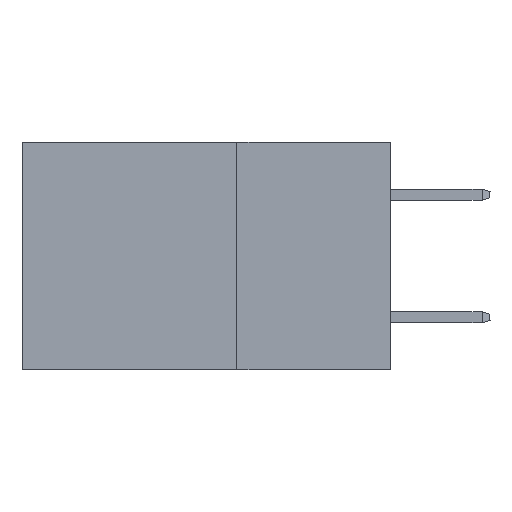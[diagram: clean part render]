
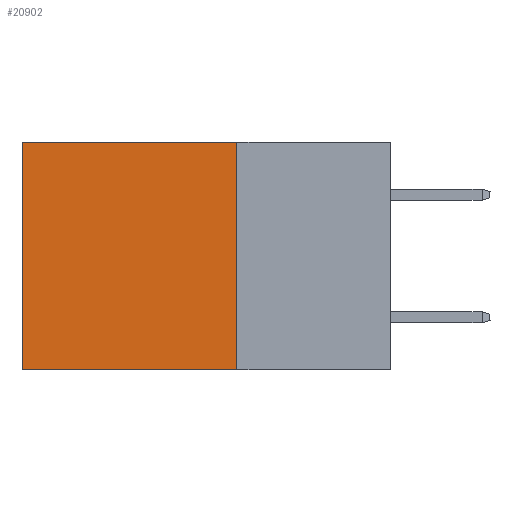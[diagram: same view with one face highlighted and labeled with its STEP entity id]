
A CAD part, left-side view. The second image highlights one B-rep face of the part: STEP entity #20902.
In plain terms, the highlighted planar face has unit normal (-1, 0, 0).
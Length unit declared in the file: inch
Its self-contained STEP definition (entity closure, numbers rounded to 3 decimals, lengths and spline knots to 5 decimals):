
#150 = CARTESIAN_POINT ( 'NONE',  ( 0.2875, 0.25, -0.37 ) ) ;
#2286 = DIRECTION ( 'NONE',  ( 0., 1., 0. ) ) ;
#2572 = DIRECTION ( 'NONE',  ( 0., 0., -1. ) ) ;
#2621 = ORIENTED_EDGE ( 'NONE', *, *, #12507, .T. ) ;
#3414 = VECTOR ( 'NONE', #31284, 39.37008 ) ;
#3448 = DIRECTION ( 'NONE',  ( 0., 0., -1. ) ) ;
#4628 = CARTESIAN_POINT ( 'NONE',  ( 0.2875, 0.6, -0.37 ) ) ;
#4707 = VECTOR ( 'NONE', #27309, 39.37008 ) ;
#4911 = VECTOR ( 'NONE', #2286, 39.37008 ) ;
#5128 = FACE_OUTER_BOUND ( 'NONE', #24840, .T. ) ;
#5456 = PLANE ( 'NONE',  #24924 ) ;
#6128 = LINE ( 'NONE', #18750, #12567 ) ;
#6677 = CARTESIAN_POINT ( 'NONE',  ( 0.2875, 0.25, -0.37 ) ) ;
#7497 = CARTESIAN_POINT ( 'NONE',  ( 0.2875, 0.25, 0. ) ) ;
#8408 = EDGE_CURVE ( 'NONE', #20372, #31596, #30320, .T. ) ;
#9521 = EDGE_CURVE ( 'NONE', #18180, #20372, #17822, .T. ) ;
#10379 = EDGE_CURVE ( 'NONE', #14375, #31596, #6128, .T. ) ;
#10787 = ORIENTED_EDGE ( 'NONE', *, *, #8408, .F. ) ;
#12507 = EDGE_CURVE ( 'NONE', #18180, #14375, #31332, .T. ) ;
#12567 = VECTOR ( 'NONE', #3448, 39.37008 ) ;
#14375 = VERTEX_POINT ( 'NONE', #32363 ) ;
#15421 = CARTESIAN_POINT ( 'NONE',  ( 0.2875, 0.25, 0. ) ) ;
#17143 = ORIENTED_EDGE ( 'NONE', *, *, #9521, .F. ) ;
#17822 = LINE ( 'NONE', #21360, #3414 ) ;
#17870 = DIRECTION ( 'NONE',  ( 1., 0., 0. ) ) ;
#18180 = VERTEX_POINT ( 'NONE', #31542 ) ;
#18750 = CARTESIAN_POINT ( 'NONE',  ( 0.2875, 0.6, 0. ) ) ;
#20372 = VERTEX_POINT ( 'NONE', #150 ) ;
#20902 = ADVANCED_FACE ( 'NONE', ( #5128 ), #5456, .F. ) ;
#21360 = CARTESIAN_POINT ( 'NONE',  ( 0.2875, 0.25, 0. ) ) ;
#24840 = EDGE_LOOP ( 'NONE', ( #27029, #10787, #17143, #2621 ) ) ;
#24924 = AXIS2_PLACEMENT_3D ( 'NONE', #7497, #17870, #2572 ) ;
#27029 = ORIENTED_EDGE ( 'NONE', *, *, #10379, .T. ) ;
#27309 = DIRECTION ( 'NONE',  ( 0., 1., 0. ) ) ;
#30320 = LINE ( 'NONE', #6677, #4707 ) ;
#31284 = DIRECTION ( 'NONE',  ( 0., 0., -1. ) ) ;
#31332 = LINE ( 'NONE', #15421, #4911 ) ;
#31542 = CARTESIAN_POINT ( 'NONE',  ( 0.2875, 0.25, 0. ) ) ;
#31596 = VERTEX_POINT ( 'NONE', #4628 ) ;
#32363 = CARTESIAN_POINT ( 'NONE',  ( 0.2875, 0.6, 0. ) ) ;
